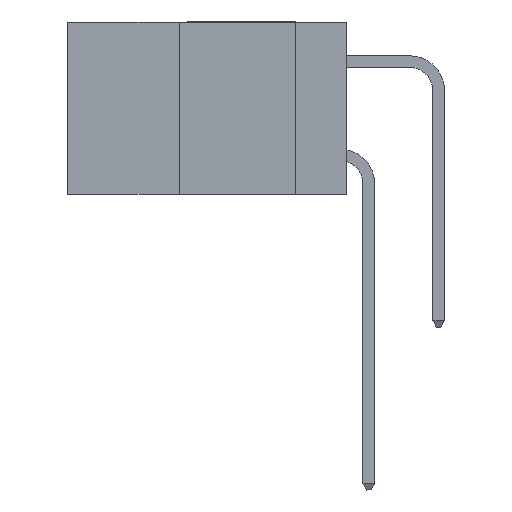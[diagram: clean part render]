
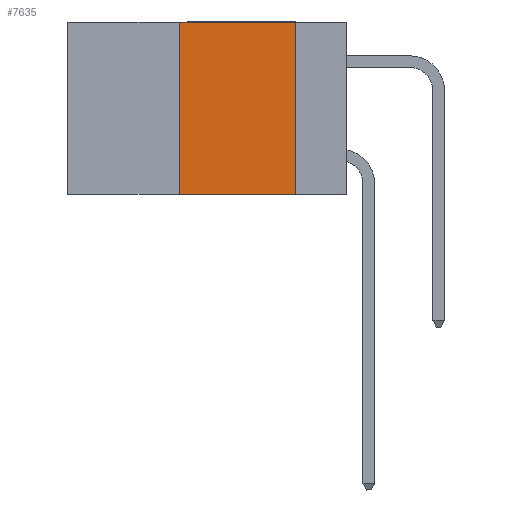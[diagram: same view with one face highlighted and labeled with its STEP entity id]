
A CAD part, left-side view. The second image highlights one B-rep face of the part: STEP entity #7635.
In plain terms, the highlighted planar face has unit normal (-1, 0, 0).
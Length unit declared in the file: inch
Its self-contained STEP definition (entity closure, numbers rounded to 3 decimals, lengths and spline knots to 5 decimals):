
#668 = CARTESIAN_POINT ( 'NONE',  ( 0., 0.36, -0.37 ) ) ;
#677 = DIRECTION ( 'NONE',  ( 0., -1., 0. ) ) ;
#756 = DIRECTION ( 'NONE',  ( 1., 0., 0. ) ) ;
#767 = CARTESIAN_POINT ( 'NONE',  ( 0., 0.36, 0. ) ) ;
#892 = FACE_OUTER_BOUND ( 'NONE', #8148, .T. ) ;
#955 = EDGE_CURVE ( 'NONE', #5176, #4562, #11824, .T. ) ;
#2730 = EDGE_CURVE ( 'NONE', #4562, #4540, #8042, .T. ) ;
#2904 = VERTEX_POINT ( 'NONE', #668 ) ;
#2908 = VECTOR ( 'NONE', #6903, 39.37008 ) ;
#4182 = CARTESIAN_POINT ( 'NONE',  ( 0., 0.11, -0.37 ) ) ;
#4540 = VERTEX_POINT ( 'NONE', #4182 ) ;
#4562 = VERTEX_POINT ( 'NONE', #8752 ) ;
#5176 = VERTEX_POINT ( 'NONE', #767 ) ;
#5351 = VECTOR ( 'NONE', #7945, 39.37008 ) ;
#5446 = PLANE ( 'NONE',  #8220 ) ;
#6164 = LINE ( 'NONE', #9003, #10674 ) ;
#6386 = DIRECTION ( 'NONE',  ( 0., -1., 0. ) ) ;
#6463 = CARTESIAN_POINT ( 'NONE',  ( 0., 0.6, 0. ) ) ;
#6903 = DIRECTION ( 'NONE',  ( 0., 0., -1. ) ) ;
#7635 = ADVANCED_FACE ( 'NONE', ( #892 ), #5446, .F. ) ;
#7777 = LINE ( 'NONE', #8815, #5351 ) ;
#7795 = CARTESIAN_POINT ( 'NONE',  ( 0., 0.11, 0. ) ) ;
#7945 = DIRECTION ( 'NONE',  ( 0., 0., 1. ) ) ;
#8002 = ORIENTED_EDGE ( 'NONE', *, *, #955, .F. ) ;
#8042 = LINE ( 'NONE', #7795, #2908 ) ;
#8148 = EDGE_LOOP ( 'NONE', ( #11306, #8002, #10331, #11480 ) ) ;
#8220 = AXIS2_PLACEMENT_3D ( 'NONE', #9950, #756, #11741 ) ;
#8752 = CARTESIAN_POINT ( 'NONE',  ( 0., 0.11, 0. ) ) ;
#8815 = CARTESIAN_POINT ( 'NONE',  ( 0., 0.36, 0. ) ) ;
#9003 = CARTESIAN_POINT ( 'NONE',  ( 0., 0.6, -0.37 ) ) ;
#9199 = VECTOR ( 'NONE', #6386, 39.37008 ) ;
#9950 = CARTESIAN_POINT ( 'NONE',  ( 0., 0.6, 0. ) ) ;
#10331 = ORIENTED_EDGE ( 'NONE', *, *, #10535, .F. ) ;
#10535 = EDGE_CURVE ( 'NONE', #2904, #5176, #7777, .T. ) ;
#10674 = VECTOR ( 'NONE', #677, 39.37008 ) ;
#11306 = ORIENTED_EDGE ( 'NONE', *, *, #2730, .F. ) ;
#11480 = ORIENTED_EDGE ( 'NONE', *, *, #11791, .T. ) ;
#11741 = DIRECTION ( 'NONE',  ( 0., 0., -1. ) ) ;
#11791 = EDGE_CURVE ( 'NONE', #2904, #4540, #6164, .T. ) ;
#11824 = LINE ( 'NONE', #6463, #9199 ) ;
